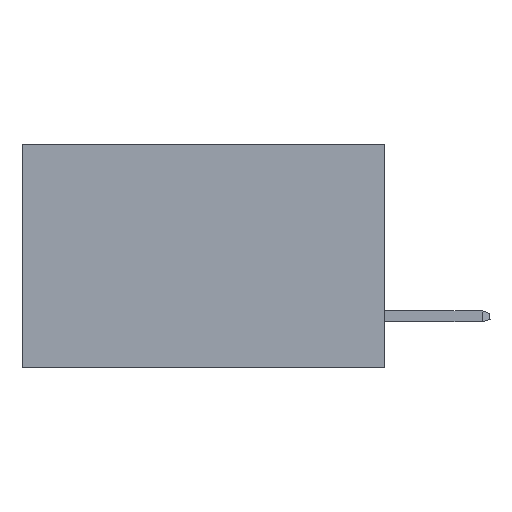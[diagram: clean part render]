
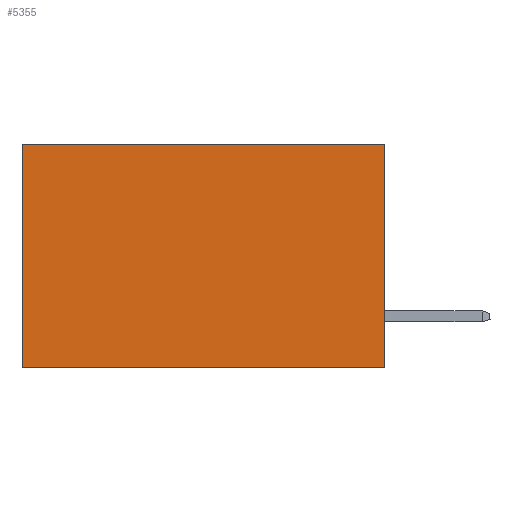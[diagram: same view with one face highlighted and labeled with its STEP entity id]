
A CAD part, left-side view. The second image highlights one B-rep face of the part: STEP entity #5355.
In plain terms, the highlighted planar face has unit normal (-1, 0, 0).
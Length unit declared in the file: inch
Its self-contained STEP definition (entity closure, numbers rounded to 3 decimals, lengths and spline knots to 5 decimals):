
#207 = PLANE ( 'NONE',  #17045 ) ;
#614 = ORIENTED_EDGE ( 'NONE', *, *, #8597, .F. ) ;
#856 = DIRECTION ( 'NONE',  ( 0., 0., -1. ) ) ;
#881 = VERTEX_POINT ( 'NONE', #9249 ) ;
#1467 = VERTEX_POINT ( 'NONE', #10897 ) ;
#1572 = CARTESIAN_POINT ( 'NONE',  ( 0.298, 0., -0.37 ) ) ;
#1740 = VECTOR ( 'NONE', #11185, 39.37008 ) ;
#2136 = VERTEX_POINT ( 'NONE', #8202 ) ;
#2338 = EDGE_CURVE ( 'NONE', #2136, #3601, #20343, .T. ) ;
#3601 = VERTEX_POINT ( 'NONE', #8570 ) ;
#3776 = LINE ( 'NONE', #16776, #17698 ) ;
#4017 = EDGE_CURVE ( 'NONE', #2136, #1467, #3776, .T. ) ;
#4944 = LINE ( 'NONE', #4947, #8153 ) ;
#4947 = CARTESIAN_POINT ( 'NONE',  ( 0.298, 0.6, 0. ) ) ;
#5355 = ADVANCED_FACE ( 'NONE', ( #14609 ), #207, .F. ) ;
#5503 = CARTESIAN_POINT ( 'NONE',  ( 0.298, 0., 0. ) ) ;
#7164 = EDGE_LOOP ( 'NONE', ( #17802, #614, #18508, #17678 ) ) ;
#8153 = VECTOR ( 'NONE', #16016, 39.37008 ) ;
#8202 = CARTESIAN_POINT ( 'NONE',  ( 0.298, 0., 0. ) ) ;
#8570 = CARTESIAN_POINT ( 'NONE',  ( 0.298, 0., -0.37 ) ) ;
#8597 = EDGE_CURVE ( 'NONE', #3601, #881, #14374, .T. ) ;
#9249 = CARTESIAN_POINT ( 'NONE',  ( 0.298, 0.6, -0.37 ) ) ;
#10897 = CARTESIAN_POINT ( 'NONE',  ( 0.298, 0.6, 0. ) ) ;
#11185 = DIRECTION ( 'NONE',  ( 0., 1., 0. ) ) ;
#11589 = CARTESIAN_POINT ( 'NONE',  ( 0.298, 0., 0. ) ) ;
#14374 = LINE ( 'NONE', #1572, #1740 ) ;
#14609 = FACE_OUTER_BOUND ( 'NONE', #7164, .T. ) ;
#16016 = DIRECTION ( 'NONE',  ( 0., 0., -1. ) ) ;
#16071 = DIRECTION ( 'NONE',  ( 1., 0., 0. ) ) ;
#16220 = DIRECTION ( 'NONE',  ( 0., 0., -1. ) ) ;
#16776 = CARTESIAN_POINT ( 'NONE',  ( 0.298, 0., 0. ) ) ;
#17045 = AXIS2_PLACEMENT_3D ( 'NONE', #11589, #16071, #16220 ) ;
#17678 = ORIENTED_EDGE ( 'NONE', *, *, #4017, .T. ) ;
#17698 = VECTOR ( 'NONE', #18251, 39.37008 ) ;
#17733 = EDGE_CURVE ( 'NONE', #1467, #881, #4944, .T. ) ;
#17802 = ORIENTED_EDGE ( 'NONE', *, *, #17733, .T. ) ;
#18251 = DIRECTION ( 'NONE',  ( 0., 1., 0. ) ) ;
#18508 = ORIENTED_EDGE ( 'NONE', *, *, #2338, .F. ) ;
#18594 = VECTOR ( 'NONE', #856, 39.37008 ) ;
#20343 = LINE ( 'NONE', #5503, #18594 ) ;
